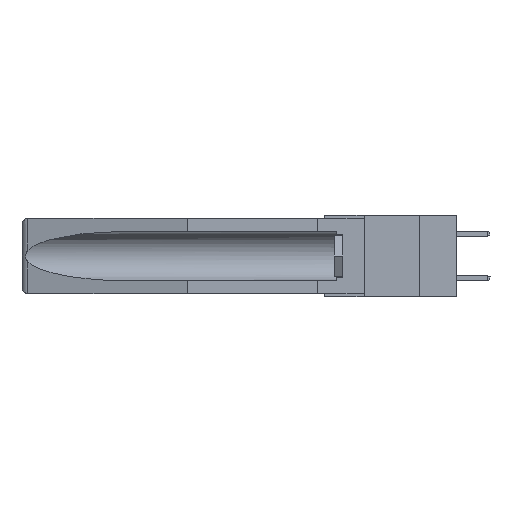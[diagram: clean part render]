
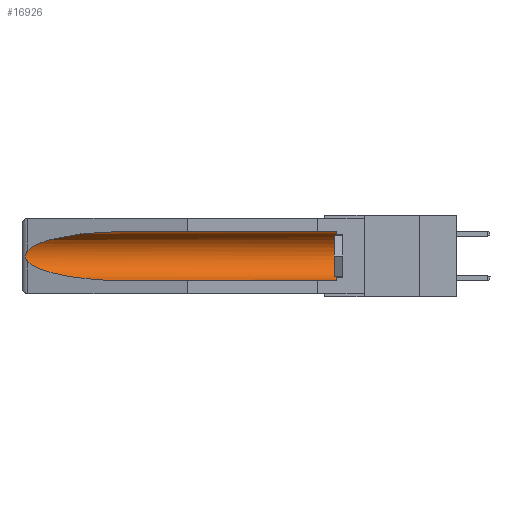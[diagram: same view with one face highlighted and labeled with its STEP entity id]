
A CAD part, left-side view. The second image highlights one B-rep face of the part: STEP entity #16926.
In plain terms, the highlighted cylindrical face has radius 2.857 mm (diameter 5.715 mm), a partial arc.
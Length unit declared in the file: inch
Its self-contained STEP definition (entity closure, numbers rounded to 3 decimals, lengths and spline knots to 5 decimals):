
#71 = CARTESIAN_POINT ( 'NONE',  ( 0.26537, 1.52718, -0.14972 ) ) ;
#81 = AXIS2_PLACEMENT_3D ( 'NONE', #308, #16052, #8219 ) ;
#139 = AXIS2_PLACEMENT_3D ( 'NONE', #15623, #11154, #15877 ) ;
#185 = VERTEX_POINT ( 'NONE', #11126 ) ;
#308 = CARTESIAN_POINT ( 'NONE',  ( 0.155, -0.30754, -0.1715 ) ) ;
#506 = VERTEX_POINT ( 'NONE', #8914 ) ;
#687 = CYLINDRICAL_SURFACE ( 'NONE', #81, 0.1125 ) ;
#916 = CARTESIAN_POINT ( 'NONE',  ( 0.25451, 1.48313, -0.09465 ) ) ;
#918 = CARTESIAN_POINT ( 'NONE',  ( 0.21114, 1.30732, -0.284 ) ) ;
#940 = FACE_OUTER_BOUND ( 'NONE', #19490, .T. ) ;
#1008 = DIRECTION ( 'NONE',  ( 0., 1., 0. ) ) ;
#1106 = ORIENTED_EDGE ( 'NONE', *, *, #12542, .T. ) ;
#1392 = CARTESIAN_POINT ( 'NONE',  ( 0.26654, 1.53092, -0.15636 ) ) ;
#2395 = B_SPLINE_CURVE_WITH_KNOTS ( 'NONE', 3,
 ( #71, #7671, #1392, #9230, #10890, #18642, #20177, #7594, #17280, #7798 ),
 .UNSPECIFIED., .F., .F.,
 ( 4, 2, 2, 2, 4 ),
 ( 0., 0.00029, 0.00058, 0.00087, 0.00117 ),
 .UNSPECIFIED. ) ;
#2526 = VERTEX_POINT ( 'NONE', #6524 ) ;
#2585 = ORIENTED_EDGE ( 'NONE', *, *, #17973, .F. ) ;
#4203 = CARTESIAN_POINT ( 'NONE',  ( 0.25451, 1.48313, -0.24835 ) ) ;
#4212 = EDGE_CURVE ( 'NONE', #2526, #506, #2395, .T. ) ;
#5098 = CARTESIAN_POINT ( 'NONE',  ( 0.155, 0.126, -0.059 ) ) ;
#5290 = DIRECTION ( 'NONE',  ( 0., 1., 0. ) ) ;
#5300 = VECTOR ( 'NONE', #5290, 39.37008 ) ;
#5723 = CARTESIAN_POINT ( 'NONE',  ( 0.155, -0.30754, -0.059 ) ) ;
#6055 = EDGE_CURVE ( 'NONE', #9792, #7025, #9977, .T. ) ;
#6524 = CARTESIAN_POINT ( 'NONE',  ( 0.26537, 1.52718, -0.14972 ) ) ;
#6922 = CARTESIAN_POINT ( 'NONE',  ( 0.155, -0.30754, -0.284 ) ) ;
#7025 = VERTEX_POINT ( 'NONE', #5098 ) ;
#7594 = CARTESIAN_POINT ( 'NONE',  ( 0.26655, 1.53094, -0.18657 ) ) ;
#7671 = CARTESIAN_POINT ( 'NONE',  ( 0.26597, 1.52961, -0.15275 ) ) ;
#7798 = CARTESIAN_POINT ( 'NONE',  ( 0.26537, 1.52718, -0.19328 ) ) ;
#8219 = DIRECTION ( 'NONE',  ( 0., 0., 1. ) ) ;
#8751 = CARTESIAN_POINT ( 'NONE',  ( 0.26537, 1.52718, -0.14972 ) ) ;
#8914 = CARTESIAN_POINT ( 'NONE',  ( 0.26537, 1.52718, -0.19328 ) ) ;
#9091 = CARTESIAN_POINT ( 'NONE',  ( 0.155, 1.07973, -0.059 ) ) ;
#9230 = CARTESIAN_POINT ( 'NONE',  ( 0.2673, 1.5327, -0.16383 ) ) ;
#9441 = LINE ( 'NONE', #6922, #5300 ) ;
#9792 = VERTEX_POINT ( 'NONE', #20209 ) ;
#9977 = CIRCLE ( 'NONE', #139, 0.1125 ) ;
#10890 = CARTESIAN_POINT ( 'NONE',  ( 0.2675, 1.53308, -0.16763 ) ) ;
#11022 = VECTOR ( 'NONE', #1008, 39.37008 ) ;
#11126 = CARTESIAN_POINT ( 'NONE',  ( 0.155, 1.07973, -0.284 ) ) ;
#11154 = DIRECTION ( 'NONE',  ( 0., -1., 0. ) ) ;
#12015 = LINE ( 'NONE', #5723, #11022 ) ;
#12542 = EDGE_CURVE ( 'NONE', #7025, #15348, #12015, .T. ) ;
#12797 = ORIENTED_EDGE ( 'NONE', *, *, #4212, .T. ) ;
#12942 = EDGE_CURVE ( 'NONE', #506, #185, #17323, .T. ) ;
#13064 = EDGE_CURVE ( 'NONE', #15348, #2526, #13671, .T. ) ;
#13089 = ORIENTED_EDGE ( 'NONE', *, *, #12942, .T. ) ;
#13152 = CARTESIAN_POINT ( 'NONE',  ( 0.155, 1.07973, -0.059 ) ) ;
#13671 =( BOUNDED_CURVE ( )  B_SPLINE_CURVE ( 3, ( #13152, #19691, #916, #8751 ),
 .UNSPECIFIED., .F., .F. ) 
 B_SPLINE_CURVE_WITH_KNOTS ( ( 4, 4 ),
 ( 4.71239, 6.08839 ),
 .UNSPECIFIED. ) 
 CURVE ( )  GEOMETRIC_REPRESENTATION_ITEM ( )  RATIONAL_B_SPLINE_CURVE ( ( 1., 0.848, 0.848, 1. ) ) 
 REPRESENTATION_ITEM ( '' )  );
#15221 = CARTESIAN_POINT ( 'NONE',  ( 0.26537, 1.52718, -0.19328 ) ) ;
#15348 = VERTEX_POINT ( 'NONE', #9091 ) ;
#15623 = CARTESIAN_POINT ( 'NONE',  ( 0.155, 0.126, -0.1715 ) ) ;
#15877 = DIRECTION ( 'NONE',  ( 0., 0., 1. ) ) ;
#16052 = DIRECTION ( 'NONE',  ( 0., 1., 0. ) ) ;
#16308 = ORIENTED_EDGE ( 'NONE', *, *, #6055, .T. ) ;
#16641 = ORIENTED_EDGE ( 'NONE', *, *, #13064, .T. ) ;
#16795 = CARTESIAN_POINT ( 'NONE',  ( 0.155, 1.07973, -0.284 ) ) ;
#16926 = ADVANCED_FACE ( 'NONE', ( #940 ), #687, .F. ) ;
#17280 = CARTESIAN_POINT ( 'NONE',  ( 0.26597, 1.5296, -0.19026 ) ) ;
#17323 =( BOUNDED_CURVE ( )  B_SPLINE_CURVE ( 3, ( #15221, #4203, #918, #16795 ),
 .UNSPECIFIED., .F., .F. ) 
 B_SPLINE_CURVE_WITH_KNOTS ( ( 4, 4 ),
 ( 0.1948, 1.5708 ),
 .UNSPECIFIED. ) 
 CURVE ( )  GEOMETRIC_REPRESENTATION_ITEM ( )  RATIONAL_B_SPLINE_CURVE ( ( 1., 0.848, 0.848, 1. ) ) 
 REPRESENTATION_ITEM ( '' )  );
#17973 = EDGE_CURVE ( 'NONE', #9792, #185, #9441, .T. ) ;
#18642 = CARTESIAN_POINT ( 'NONE',  ( 0.2675, 1.53308, -0.17534 ) ) ;
#19490 = EDGE_LOOP ( 'NONE', ( #16641, #12797, #13089, #2585, #16308, #1106 ) ) ;
#19691 = CARTESIAN_POINT ( 'NONE',  ( 0.21114, 1.30732, -0.059 ) ) ;
#20177 = CARTESIAN_POINT ( 'NONE',  ( 0.2673, 1.53269, -0.17917 ) ) ;
#20209 = CARTESIAN_POINT ( 'NONE',  ( 0.155, 0.126, -0.284 ) ) ;
